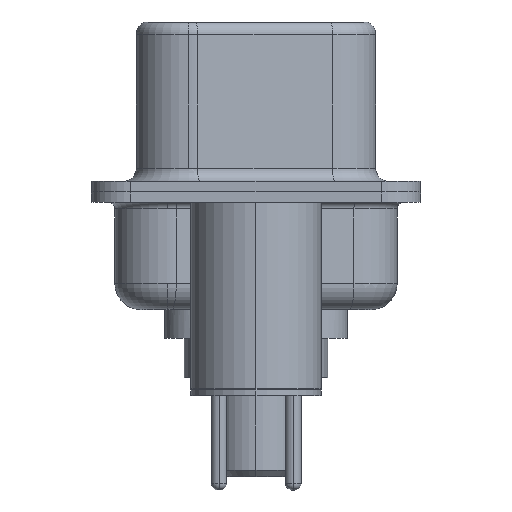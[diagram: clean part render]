
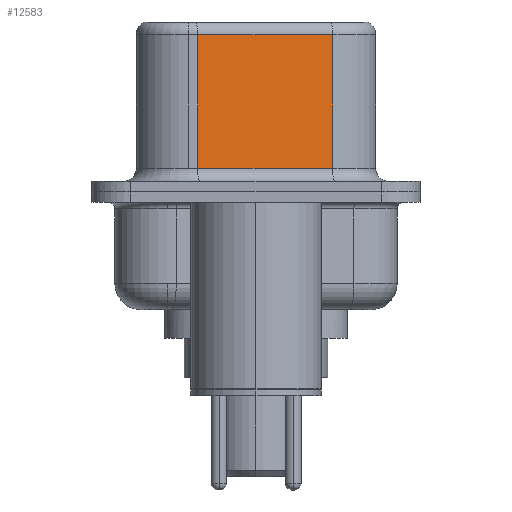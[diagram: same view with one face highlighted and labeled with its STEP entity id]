
A CAD part, left-side view. The second image highlights one B-rep face of the part: STEP entity #12583.
In plain terms, the highlighted planar face has unit normal (-0.985, -0.174, 0).
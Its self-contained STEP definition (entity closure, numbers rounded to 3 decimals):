
#111 = VERTEX_POINT ( 'NONE', #12822 ) ;
#605 = ORIENTED_EDGE ( 'NONE', *, *, #5081, .T. ) ;
#627 = CARTESIAN_POINT ( 'NONE',  ( 4.565, -2.927, 6.52 ) ) ;
#1217 = FACE_OUTER_BOUND ( 'NONE', #4074, .T. ) ;
#1609 = VECTOR ( 'NONE', #4782, 1000. ) ;
#1793 = CARTESIAN_POINT ( 'NONE',  ( 4.565, -2.927, 0.9 ) ) ;
#1999 = CARTESIAN_POINT ( 'NONE',  ( 4.565, -2.927, 6.02 ) ) ;
#3796 = CARTESIAN_POINT ( 'NONE',  ( 4.565, -2.927, 6.02 ) ) ;
#3986 = VERTEX_POINT ( 'NONE', #16501 ) ;
#4074 = EDGE_LOOP ( 'NONE', ( #11890, #4454, #12129, #605 ) ) ;
#4454 = ORIENTED_EDGE ( 'NONE', *, *, #16847, .T. ) ;
#4700 = DIRECTION ( 'NONE',  ( 0.985, 0.174, 0. ) ) ;
#4782 = DIRECTION ( 'NONE',  ( 0., 0., -1. ) ) ;
#5081 = EDGE_CURVE ( 'NONE', #3986, #5674, #13510, .T. ) ;
#5656 = EDGE_CURVE ( 'NONE', #16298, #5674, #11664, .T. ) ;
#5674 = VERTEX_POINT ( 'NONE', #15660 ) ;
#5699 = VECTOR ( 'NONE', #16451, 1000. ) ;
#8104 = LINE ( 'NONE', #10380, #1609 ) ;
#8388 = VECTOR ( 'NONE', #10806, 1000. ) ;
#10380 = CARTESIAN_POINT ( 'NONE',  ( 3.655, 2.233, 6.52 ) ) ;
#10729 = AXIS2_PLACEMENT_3D ( 'NONE', #627, #4700, #14379 ) ;
#10806 = DIRECTION ( 'NONE',  ( 0., 0., -1. ) ) ;
#11664 = LINE ( 'NONE', #15426, #8388 ) ;
#11692 = PLANE ( 'NONE',  #10729 ) ;
#11758 = DIRECTION ( 'NONE',  ( -0.174, 0.985, 0. ) ) ;
#11890 = ORIENTED_EDGE ( 'NONE', *, *, #5656, .F. ) ;
#12129 = ORIENTED_EDGE ( 'NONE', *, *, #14108, .T. ) ;
#12550 = LINE ( 'NONE', #1999, #15695 ) ;
#12583 = ADVANCED_FACE ( 'NONE', ( #1217 ), #11692, .F. ) ;
#12822 = CARTESIAN_POINT ( 'NONE',  ( 3.655, 2.233, 6.02 ) ) ;
#13510 = LINE ( 'NONE', #1793, #5699 ) ;
#14108 = EDGE_CURVE ( 'NONE', #111, #3986, #8104, .T. ) ;
#14379 = DIRECTION ( 'NONE',  ( -0.174, 0.985, 0. ) ) ;
#15426 = CARTESIAN_POINT ( 'NONE',  ( 4.565, -2.927, 6.52 ) ) ;
#15660 = CARTESIAN_POINT ( 'NONE',  ( 4.565, -2.927, 0.9 ) ) ;
#15695 = VECTOR ( 'NONE', #11758, 1000. ) ;
#16298 = VERTEX_POINT ( 'NONE', #3796 ) ;
#16451 = DIRECTION ( 'NONE',  ( 0.174, -0.985, 0. ) ) ;
#16501 = CARTESIAN_POINT ( 'NONE',  ( 3.655, 2.233, 0.9 ) ) ;
#16847 = EDGE_CURVE ( 'NONE', #16298, #111, #12550, .T. ) ;
